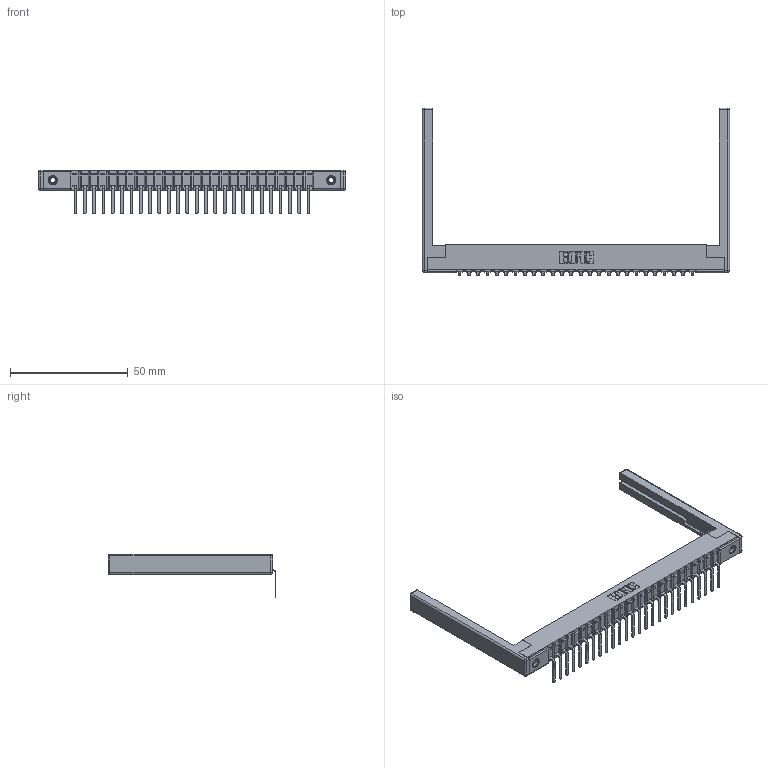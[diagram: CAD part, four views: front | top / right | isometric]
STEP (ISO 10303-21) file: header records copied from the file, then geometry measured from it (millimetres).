
FILE_DESCRIPTION (( 'STEP AP203' ), '1' );
FILE_NAME ('307-026-557-168.STEP', '2019-09-05T02:20:12', ( '' ), ( '' ), 'SwSTEP 2.0', 'SolidWorks 2016', '' );
FILE_SCHEMA (( 'CONFIG_CONTROL_DESIGN' ));
Length unit declared in the file: inch
Products named in the file (5): 307-220-068; 307-290-002_557; 307 Part_.156 Dia Mounting Holes; 345-250-001_345-250-001-102; 307-026-557-168
Assembly tree (31 placements, depth 2):
  307-026-557-168
    307 Part_.156 Dia Mounting Holes
    307-290-002_557  x26
    307-220-068  x2
    345-250-001_345-250-001-102  x2
Bounding box: 130.45 x 71.29 x 18.67 mm (x, y, z)
Volume: 13243.4 mm3; surface area: 20467.5 mm2
Topology: 31 solids, 31 shells, 2327 faces, 7057 edges, 4610 vertices
Faces by surface type: plane 1380, cylinder 869, sphere 62, cone 12, torus 4
Entity records: 27875 total; most frequent: CARTESIAN_POINT 4665, ORIENTED_EDGE 4644, DIRECTION 4558, EDGE_CURVE 2322, VECTOR 1768, LINE 1768, VERTEX_POINT 1502, AXIS2_PLACEMENT_3D 1395
